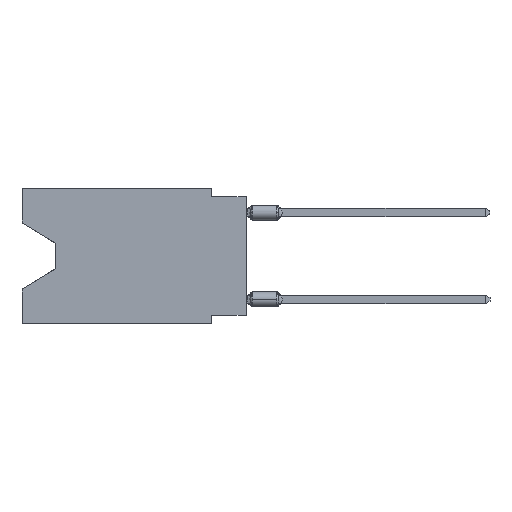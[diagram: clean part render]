
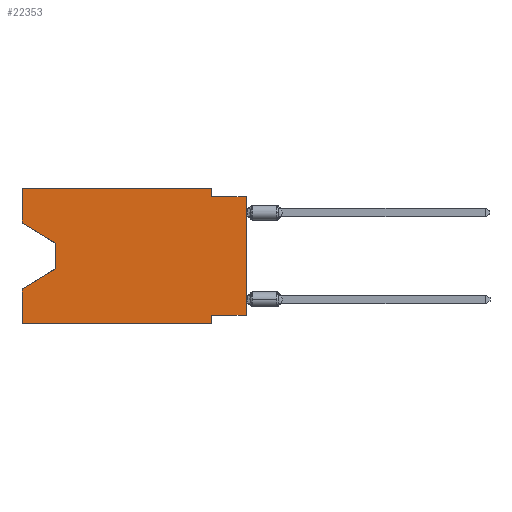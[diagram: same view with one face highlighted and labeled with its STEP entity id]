
A CAD part, left-side view. The second image highlights one B-rep face of the part: STEP entity #22353.
In plain terms, the highlighted planar face has unit normal (-1, 0, 0).
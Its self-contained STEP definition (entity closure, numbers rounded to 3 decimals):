
#34 = PLANE ( 'NONE',  #1343 ) ;
#173 = EDGE_CURVE ( 'NONE', #4670, #850, #15310, .T. ) ;
#362 = VERTEX_POINT ( 'NONE', #21183 ) ;
#517 = CARTESIAN_POINT ( 'NONE',  ( 0., 13.97, -4.013 ) ) ;
#630 = EDGE_CURVE ( 'NONE', #3635, #6330, #10523, .T. ) ;
#812 = VECTOR ( 'NONE', #3253, 1000. ) ;
#850 = VERTEX_POINT ( 'NONE', #21610 ) ;
#1092 = VERTEX_POINT ( 'NONE', #22298 ) ;
#1343 = AXIS2_PLACEMENT_3D ( 'NONE', #7064, #19526, #3736 ) ;
#1407 = CARTESIAN_POINT ( 'NONE',  ( 0., 16.383, -2.546 ) ) ;
#1567 = VERTEX_POINT ( 'NONE', #8869 ) ;
#2055 = LINE ( 'NONE', #15879, #5216 ) ;
#2238 = ORIENTED_EDGE ( 'NONE', *, *, #6046, .T. ) ;
#2589 = EDGE_CURVE ( 'NONE', #4670, #362, #4143, .T. ) ;
#2887 = CARTESIAN_POINT ( 'NONE',  ( 0., 16.383, -2.546 ) ) ;
#3012 = VECTOR ( 'NONE', #19601, 1000. ) ;
#3034 = LINE ( 'NONE', #22508, #3012 ) ;
#3151 = EDGE_CURVE ( 'NONE', #15615, #3635, #15158, .T. ) ;
#3235 = ORIENTED_EDGE ( 'NONE', *, *, #630, .F. ) ;
#3253 = DIRECTION ( 'NONE',  ( 0., 0., -1. ) ) ;
#3283 = DIRECTION ( 'NONE',  ( 0., 0., 1. ) ) ;
#3362 = LINE ( 'NONE', #1407, #18497 ) ;
#3411 = ORIENTED_EDGE ( 'NONE', *, *, #14118, .T. ) ;
#3456 = CARTESIAN_POINT ( 'NONE',  ( 0., 2.54, -9.906 ) ) ;
#3613 = CARTESIAN_POINT ( 'NONE',  ( 0., 13.97, -5.893 ) ) ;
#3635 = VERTEX_POINT ( 'NONE', #5201 ) ;
#3736 = DIRECTION ( 'NONE',  ( 0., 0., -1. ) ) ;
#3757 = ORIENTED_EDGE ( 'NONE', *, *, #6907, .F. ) ;
#4143 = LINE ( 'NONE', #11138, #16226 ) ;
#4256 = DIRECTION ( 'NONE',  ( 0., -1., 0. ) ) ;
#4670 = VERTEX_POINT ( 'NONE', #16518 ) ;
#5149 = CARTESIAN_POINT ( 'NONE',  ( 0., 16.383, 0. ) ) ;
#5201 = CARTESIAN_POINT ( 'NONE',  ( 0., 16.383, 0. ) ) ;
#5216 = VECTOR ( 'NONE', #17750, 1000. ) ;
#5238 = FACE_OUTER_BOUND ( 'NONE', #20672, .T. ) ;
#5430 = EDGE_CURVE ( 'NONE', #6330, #19519, #20951, .T. ) ;
#6030 = ORIENTED_EDGE ( 'NONE', *, *, #3151, .F. ) ;
#6046 = EDGE_CURVE ( 'NONE', #1092, #8813, #20904, .T. ) ;
#6330 = VERTEX_POINT ( 'NONE', #22164 ) ;
#6555 = VECTOR ( 'NONE', #3283, 1000. ) ;
#6907 = EDGE_CURVE ( 'NONE', #1567, #362, #15431, .T. ) ;
#6933 = CARTESIAN_POINT ( 'NONE',  ( 0., 13.97, -4.013 ) ) ;
#7064 = CARTESIAN_POINT ( 'NONE',  ( 0., 16.383, 0. ) ) ;
#7551 = VECTOR ( 'NONE', #10221, 1000. ) ;
#7980 = ORIENTED_EDGE ( 'NONE', *, *, #173, .F. ) ;
#8057 = CARTESIAN_POINT ( 'NONE',  ( 0., 0., -0.635 ) ) ;
#8813 = VERTEX_POINT ( 'NONE', #19569 ) ;
#8869 = CARTESIAN_POINT ( 'NONE',  ( 0., 2.54, -9.271 ) ) ;
#8941 = DIRECTION ( 'NONE',  ( 0., 0., -1. ) ) ;
#9466 = EDGE_CURVE ( 'NONE', #1092, #1567, #3034, .T. ) ;
#10058 = VERTEX_POINT ( 'NONE', #3613 ) ;
#10221 = DIRECTION ( 'NONE',  ( 0., 0., -1. ) ) ;
#10523 = LINE ( 'NONE', #5149, #16907 ) ;
#10597 = VECTOR ( 'NONE', #13588, 1000. ) ;
#10686 = VECTOR ( 'NONE', #20575, 1000. ) ;
#10846 = ORIENTED_EDGE ( 'NONE', *, *, #14151, .T. ) ;
#10874 = ORIENTED_EDGE ( 'NONE', *, *, #5430, .F. ) ;
#11138 = CARTESIAN_POINT ( 'NONE',  ( 0., 16.383, -9.906 ) ) ;
#11720 = ORIENTED_EDGE ( 'NONE', *, *, #9466, .F. ) ;
#11790 = ORIENTED_EDGE ( 'NONE', *, *, #13303, .T. ) ;
#11800 = DIRECTION ( 'NONE',  ( 0., -1., 0. ) ) ;
#12100 = VERTEX_POINT ( 'NONE', #517 ) ;
#12207 = ORIENTED_EDGE ( 'NONE', *, *, #2589, .T. ) ;
#12218 = DIRECTION ( 'NONE',  ( 0., -0.855, -0.519 ) ) ;
#12809 = EDGE_CURVE ( 'NONE', #19519, #8813, #22607, .T. ) ;
#13000 = ORIENTED_EDGE ( 'NONE', *, *, #12809, .F. ) ;
#13303 = EDGE_CURVE ( 'NONE', #10058, #850, #2055, .T. ) ;
#13588 = DIRECTION ( 'NONE',  ( 0., 0., 1. ) ) ;
#13874 = CARTESIAN_POINT ( 'NONE',  ( 0., 0., 0. ) ) ;
#14118 = EDGE_CURVE ( 'NONE', #12100, #10058, #17559, .T. ) ;
#14151 = EDGE_CURVE ( 'NONE', #15615, #12100, #3362, .T. ) ;
#14494 = VECTOR ( 'NONE', #15109, 1000. ) ;
#15109 = DIRECTION ( 'NONE',  ( 0., -1., 0. ) ) ;
#15158 = LINE ( 'NONE', #21970, #10686 ) ;
#15310 = LINE ( 'NONE', #22360, #10597 ) ;
#15431 = LINE ( 'NONE', #3456, #7551 ) ;
#15615 = VERTEX_POINT ( 'NONE', #2887 ) ;
#15879 = CARTESIAN_POINT ( 'NONE',  ( 0., 13.97, -5.893 ) ) ;
#16226 = VECTOR ( 'NONE', #4256, 1000. ) ;
#16518 = CARTESIAN_POINT ( 'NONE',  ( 0., 16.383, -9.906 ) ) ;
#16907 = VECTOR ( 'NONE', #11800, 1000. ) ;
#17559 = LINE ( 'NONE', #6933, #812 ) ;
#17750 = DIRECTION ( 'NONE',  ( 0., 0.855, -0.519 ) ) ;
#18497 = VECTOR ( 'NONE', #12218, 1000. ) ;
#19519 = VERTEX_POINT ( 'NONE', #21100 ) ;
#19526 = DIRECTION ( 'NONE',  ( 1., 0., 0. ) ) ;
#19569 = CARTESIAN_POINT ( 'NONE',  ( 0., 0., -0.635 ) ) ;
#19601 = DIRECTION ( 'NONE',  ( 0., 1., 0. ) ) ;
#20575 = DIRECTION ( 'NONE',  ( 0., 0., 1. ) ) ;
#20672 = EDGE_LOOP ( 'NONE', ( #10846, #3411, #11790, #7980, #12207, #3757, #11720, #2238, #13000, #10874, #3235, #6030 ) ) ;
#20885 = VECTOR ( 'NONE', #8941, 1000. ) ;
#20904 = LINE ( 'NONE', #13874, #6555 ) ;
#20951 = LINE ( 'NONE', #21065, #20885 ) ;
#21065 = CARTESIAN_POINT ( 'NONE',  ( 0., 2.54, 0. ) ) ;
#21100 = CARTESIAN_POINT ( 'NONE',  ( 0., 2.54, -0.635 ) ) ;
#21183 = CARTESIAN_POINT ( 'NONE',  ( 0., 2.54, -9.906 ) ) ;
#21610 = CARTESIAN_POINT ( 'NONE',  ( 0., 16.383, -7.36 ) ) ;
#21970 = CARTESIAN_POINT ( 'NONE',  ( 0., 16.383, 0. ) ) ;
#22164 = CARTESIAN_POINT ( 'NONE',  ( 0., 2.54, 0. ) ) ;
#22298 = CARTESIAN_POINT ( 'NONE',  ( 0., 0., -9.271 ) ) ;
#22353 = ADVANCED_FACE ( 'NONE', ( #5238 ), #34, .F. ) ;
#22360 = CARTESIAN_POINT ( 'NONE',  ( 0., 16.383, 0. ) ) ;
#22508 = CARTESIAN_POINT ( 'NONE',  ( 0., 0., -9.271 ) ) ;
#22607 = LINE ( 'NONE', #8057, #14494 ) ;
